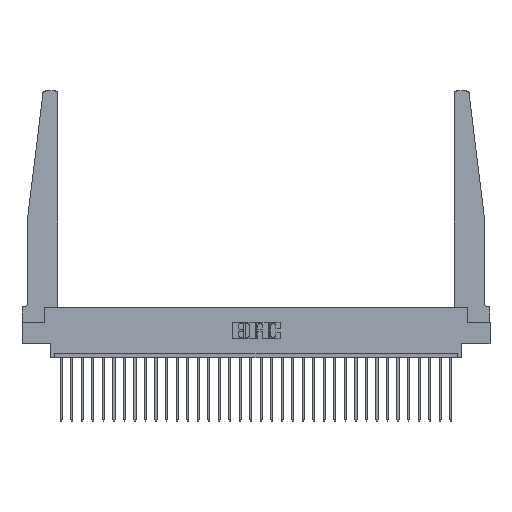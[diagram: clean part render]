
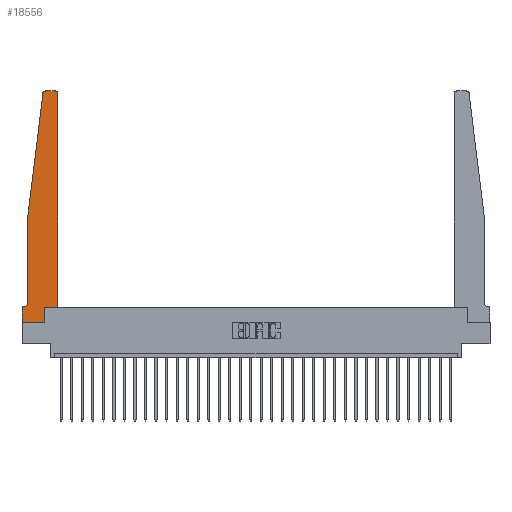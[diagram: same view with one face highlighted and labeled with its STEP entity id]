
A CAD part, top view. The second image highlights one B-rep face of the part: STEP entity #18556.
In plain terms, the highlighted planar face has unit normal (0, 0, 1).
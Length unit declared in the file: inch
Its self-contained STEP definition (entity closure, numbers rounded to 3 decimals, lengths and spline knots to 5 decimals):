
#54 = VECTOR ( 'NONE', #1165, 39.37008 ) ;
#166 = ORIENTED_EDGE ( 'NONE', *, *, #27110, .T. ) ;
#672 = CARTESIAN_POINT ( 'NONE',  ( 0.27653, 2.72, 0.37 ) ) ;
#884 = ORIENTED_EDGE ( 'NONE', *, *, #25058, .T. ) ;
#1107 = DIRECTION ( 'NONE',  ( -0.122, -0.992, 0. ) ) ;
#1165 = DIRECTION ( 'NONE',  ( 1., 0., 0. ) ) ;
#1211 = EDGE_CURVE ( 'NONE', #23220, #10180, #5576, .T. ) ;
#1637 = EDGE_CURVE ( 'NONE', #8662, #6509, #2767, .T. ) ;
#1729 = EDGE_CURVE ( 'NONE', #20146, #7498, #28403, .T. ) ;
#2267 = VERTEX_POINT ( 'NONE', #2649 ) ;
#2330 = PLANE ( 'NONE',  #14664 ) ;
#2391 = CARTESIAN_POINT ( 'NONE',  ( 0., 0., 0.37 ) ) ;
#2649 = CARTESIAN_POINT ( 'NONE',  ( 0., 0.1875, 0.37 ) ) ;
#2767 = CIRCLE ( 'NONE', #25886, 0.03 ) ;
#2858 = VECTOR ( 'NONE', #21088, 39.37008 ) ;
#2958 = DIRECTION ( 'NONE',  ( 1., 0., 0. ) ) ;
#3027 = EDGE_CURVE ( 'NONE', #6509, #8198, #24799, .T. ) ;
#3297 = AXIS2_PLACEMENT_3D ( 'NONE', #11177, #6752, #15832 ) ;
#3335 = ORIENTED_EDGE ( 'NONE', *, *, #16087, .T. ) ;
#3502 = EDGE_CURVE ( 'NONE', #7498, #2267, #27206, .T. ) ;
#3563 = CARTESIAN_POINT ( 'NONE',  ( 0.2605, 0.18, 0.37 ) ) ;
#4041 = ORIENTED_EDGE ( 'NONE', *, *, #24672, .T. ) ;
#4557 = CARTESIAN_POINT ( 'NONE',  ( 0.25, 2.75, 0.37 ) ) ;
#5452 = ORIENTED_EDGE ( 'NONE', *, *, #6410, .T. ) ;
#5576 = LINE ( 'NONE', #19987, #28773 ) ;
#5795 = LINE ( 'NONE', #2391, #27191 ) ;
#6152 = FACE_OUTER_BOUND ( 'NONE', #6695, .T. ) ;
#6410 = EDGE_CURVE ( 'NONE', #25477, #8662, #23629, .T. ) ;
#6485 = DIRECTION ( 'NONE',  ( 0., 1., 0. ) ) ;
#6509 = VERTEX_POINT ( 'NONE', #12355 ) ;
#6695 = EDGE_LOOP ( 'NONE', ( #5452, #24385, #17525, #22850, #13634, #8520, #3335, #166, #22514, #11108, #884, #4041 ) ) ;
#6752 = DIRECTION ( 'NONE',  ( 0., 0., -1. ) ) ;
#6771 = DIRECTION ( 'NONE',  ( 1., 0., 0. ) ) ;
#7021 = LINE ( 'NONE', #10315, #54 ) ;
#7498 = VERTEX_POINT ( 'NONE', #9049 ) ;
#8198 = VERTEX_POINT ( 'NONE', #19657 ) ;
#8361 = CIRCLE ( 'NONE', #24673, 0.03 ) ;
#8520 = ORIENTED_EDGE ( 'NONE', *, *, #3502, .T. ) ;
#8662 = VERTEX_POINT ( 'NONE', #19874 ) ;
#8809 = VERTEX_POINT ( 'NONE', #25222 ) ;
#9049 = CARTESIAN_POINT ( 'NONE',  ( 0.015, 0.1875, 0.37 ) ) ;
#9153 = DIRECTION ( 'NONE',  ( 0., 0., 1. ) ) ;
#10041 = LINE ( 'NONE', #11225, #25864 ) ;
#10128 = LINE ( 'NONE', #28051, #15439 ) ;
#10180 = VERTEX_POINT ( 'NONE', #3563 ) ;
#10256 = CARTESIAN_POINT ( 'NONE',  ( 0., 0., 0.37 ) ) ;
#10315 = CARTESIAN_POINT ( 'NONE',  ( 0.425, 0.18, 0.37 ) ) ;
#10633 = DIRECTION ( 'NONE',  ( 0., 0., 1. ) ) ;
#10714 = VECTOR ( 'NONE', #25284, 39.37008 ) ;
#10866 = CARTESIAN_POINT ( 'NONE',  ( 0.425, 0.18, 0.37 ) ) ;
#11108 = ORIENTED_EDGE ( 'NONE', *, *, #23459, .T. ) ;
#11177 = CARTESIAN_POINT ( 'NONE',  ( 0.015, 0.2375, 0.37 ) ) ;
#11225 = CARTESIAN_POINT ( 'NONE',  ( 0.065, 1.25, 0.37 ) ) ;
#12167 = VERTEX_POINT ( 'NONE', #21985 ) ;
#12254 = DIRECTION ( 'NONE',  ( 0., 1., 0. ) ) ;
#12355 = CARTESIAN_POINT ( 'NONE',  ( 0.24675, 2.72367, 0.37 ) ) ;
#13236 = VECTOR ( 'NONE', #21105, 39.37008 ) ;
#13634 = ORIENTED_EDGE ( 'NONE', *, *, #1729, .T. ) ;
#14344 = CARTESIAN_POINT ( 'NONE',  ( 0.065, 1.25, 0.37 ) ) ;
#14374 = CARTESIAN_POINT ( 'NONE',  ( 0.395, 2.75, 0.37 ) ) ;
#14664 = AXIS2_PLACEMENT_3D ( 'NONE', #27123, #9153, #20392 ) ;
#15439 = VECTOR ( 'NONE', #12254, 39.37008 ) ;
#15832 = DIRECTION ( 'NONE',  ( -1., 0., 0. ) ) ;
#16087 = EDGE_CURVE ( 'NONE', #2267, #12167, #20252, .T. ) ;
#17203 = VERTEX_POINT ( 'NONE', #10866 ) ;
#17525 = ORIENTED_EDGE ( 'NONE', *, *, #3027, .T. ) ;
#17806 = CARTESIAN_POINT ( 'NONE',  ( 0.395, 2.72, 0.37 ) ) ;
#18039 = DIRECTION ( 'NONE',  ( 0., -1., 0. ) ) ;
#18302 = CARTESIAN_POINT ( 'NONE',  ( 0.065, 0.2375, 0.37 ) ) ;
#18556 = ADVANCED_FACE ( 'NONE', ( #6152 ), #2330, .T. ) ;
#19657 = CARTESIAN_POINT ( 'NONE',  ( 0.065, 1.25, 0.37 ) ) ;
#19874 = CARTESIAN_POINT ( 'NONE',  ( 0.27653, 2.75, 0.37 ) ) ;
#19987 = CARTESIAN_POINT ( 'NONE',  ( 0.2605, 0.18, 0.37 ) ) ;
#20146 = VERTEX_POINT ( 'NONE', #18302 ) ;
#20252 = LINE ( 'NONE', #10256, #13236 ) ;
#20392 = DIRECTION ( 'NONE',  ( 1., 0., 0. ) ) ;
#21088 = DIRECTION ( 'NONE',  ( -1., 0., 0. ) ) ;
#21105 = DIRECTION ( 'NONE',  ( 0., -1., 0. ) ) ;
#21985 = CARTESIAN_POINT ( 'NONE',  ( 0., 0., 0.37 ) ) ;
#22514 = ORIENTED_EDGE ( 'NONE', *, *, #1211, .T. ) ;
#22850 = ORIENTED_EDGE ( 'NONE', *, *, #26412, .T. ) ;
#22959 = CARTESIAN_POINT ( 'NONE',  ( 0.065, 0.1875, 0.37 ) ) ;
#23220 = VERTEX_POINT ( 'NONE', #23465 ) ;
#23459 = EDGE_CURVE ( 'NONE', #10180, #17203, #7021, .T. ) ;
#23465 = CARTESIAN_POINT ( 'NONE',  ( 0.2605, 0., 0.37 ) ) ;
#23629 = LINE ( 'NONE', #4557, #2858 ) ;
#24385 = ORIENTED_EDGE ( 'NONE', *, *, #1637, .T. ) ;
#24672 = EDGE_CURVE ( 'NONE', #8809, #25477, #8361, .T. ) ;
#24673 = AXIS2_PLACEMENT_3D ( 'NONE', #17806, #10633, #27596 ) ;
#24799 = LINE ( 'NONE', #14344, #25157 ) ;
#25058 = EDGE_CURVE ( 'NONE', #17203, #8809, #10128, .T. ) ;
#25157 = VECTOR ( 'NONE', #1107, 39.37008 ) ;
#25222 = CARTESIAN_POINT ( 'NONE',  ( 0.425, 2.72, 0.37 ) ) ;
#25243 = DIRECTION ( 'NONE',  ( 0., 0., 1. ) ) ;
#25284 = DIRECTION ( 'NONE',  ( -1., 0., 0. ) ) ;
#25477 = VERTEX_POINT ( 'NONE', #14374 ) ;
#25864 = VECTOR ( 'NONE', #18039, 39.37008 ) ;
#25886 = AXIS2_PLACEMENT_3D ( 'NONE', #672, #25243, #2958 ) ;
#26412 = EDGE_CURVE ( 'NONE', #8198, #20146, #10041, .T. ) ;
#27110 = EDGE_CURVE ( 'NONE', #12167, #23220, #5795, .T. ) ;
#27123 = CARTESIAN_POINT ( 'NONE',  ( 0., 0.1875, 0.37 ) ) ;
#27191 = VECTOR ( 'NONE', #6771, 39.37008 ) ;
#27206 = LINE ( 'NONE', #22959, #10714 ) ;
#27596 = DIRECTION ( 'NONE',  ( 1., 0., 0. ) ) ;
#28051 = CARTESIAN_POINT ( 'NONE',  ( 0.425, 0.18, 0.37 ) ) ;
#28403 = CIRCLE ( 'NONE', #3297, 0.05 ) ;
#28773 = VECTOR ( 'NONE', #6485, 39.37008 ) ;
